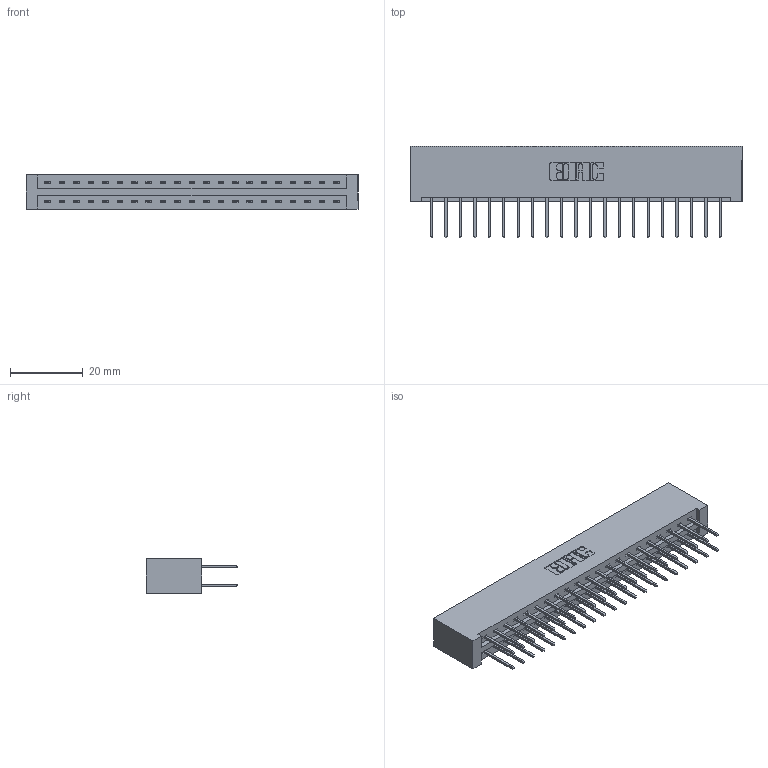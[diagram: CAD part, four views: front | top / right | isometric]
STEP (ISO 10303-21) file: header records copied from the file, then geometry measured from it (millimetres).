
FILE_DESCRIPTION (( 'STEP AP203' ), '1' );
FILE_NAME ('387-042-523-201.STEP', '2018-09-19T21:55:32', ( '' ), ( '' ), 'SwSTEP 2.0', 'SolidWorks 2016', '' );
FILE_SCHEMA (( 'CONFIG_CONTROL_DESIGN' ));
Length unit declared in the file: inch
Products named in the file (3): 337 Part_No Mounting Lugs; 345-292-001_345-293-123; 387-042-523-201
Assembly tree (43 placements, depth 2):
  387-042-523-201
    337 Part_No Mounting Lugs
    345-292-001_345-293-123  x42
Bounding box: 91.08 x 25.15 x 9.4 mm (x, y, z)
Volume: 10166.5 mm3; surface area: 11754.5 mm2
Topology: 43 solids, 43 shells, 2374 faces, 7049 edges, 4642 vertices
Faces by surface type: plane 1662, cylinder 712
Entity records: 18739 total; most frequent: CARTESIAN_POINT 3174, ORIENTED_EDGE 3110, DIRECTION 2731, EDGE_CURVE 1555, LINE 1435, VECTOR 1435, VERTEX_POINT 1034, AXIS2_PLACEMENT_3D 648
